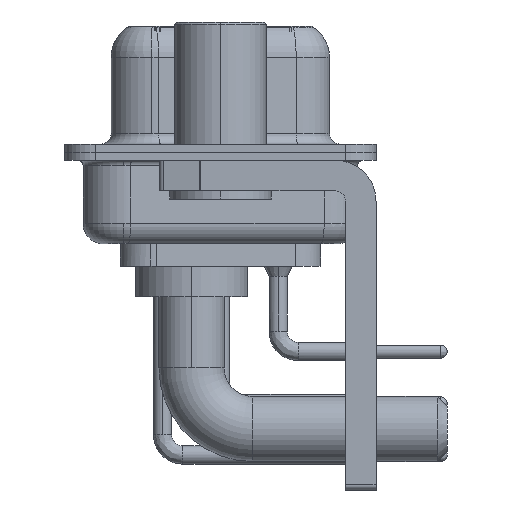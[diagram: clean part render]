
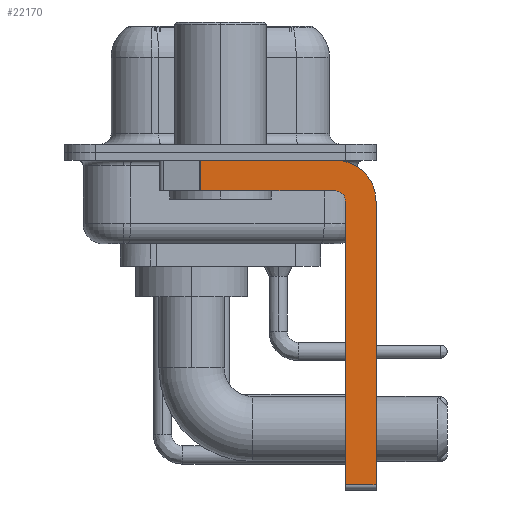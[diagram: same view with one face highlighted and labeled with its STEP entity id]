
A CAD part, left-side view. The second image highlights one B-rep face of the part: STEP entity #22170.
In plain terms, the highlighted planar face has unit normal (-1, 0, 0).
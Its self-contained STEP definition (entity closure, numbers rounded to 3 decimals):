
#495 = FACE_OUTER_BOUND ( 'NONE', #18113, .T. ) ;
#679 = DIRECTION ( 'NONE',  ( 0., 0., 1. ) ) ;
#1020 = LINE ( 'NONE', #28856, #26180 ) ;
#1079 = CARTESIAN_POINT ( 'NONE',  ( -2.9, -6.15, -16.6 ) ) ;
#1537 = DIRECTION ( 'NONE',  ( 0., 1., 0. ) ) ;
#1551 = DIRECTION ( 'NONE',  ( 1., 0., 0. ) ) ;
#1914 = DIRECTION ( 'NONE',  ( 0., 0., -1. ) ) ;
#1986 = ORIENTED_EDGE ( 'NONE', *, *, #17445, .F. ) ;
#2511 = CARTESIAN_POINT ( 'NONE',  ( -2.9, -5.65, -0.4 ) ) ;
#2996 = CARTESIAN_POINT ( 'NONE',  ( -2.9, 0.978, -1.9 ) ) ;
#3268 = VERTEX_POINT ( 'NONE', #34301 ) ;
#3313 = VERTEX_POINT ( 'NONE', #23075 ) ;
#3329 = CARTESIAN_POINT ( 'NONE',  ( -2.9, -6.15, -2.4 ) ) ;
#3332 = VECTOR ( 'NONE', #27077, 1000. ) ;
#3419 = VERTEX_POINT ( 'NONE', #7307 ) ;
#3896 = EDGE_CURVE ( 'NONE', #22963, #13782, #33438, .T. ) ;
#4553 = EDGE_CURVE ( 'NONE', #12942, #3419, #22404, .T. ) ;
#6083 = ORIENTED_EDGE ( 'NONE', *, *, #23129, .F. ) ;
#6732 = DIRECTION ( 'NONE',  ( 0., -1., 0. ) ) ;
#7307 = CARTESIAN_POINT ( 'NONE',  ( -2.9, -7.65, -16.35 ) ) ;
#7555 = ORIENTED_EDGE ( 'NONE', *, *, #3896, .T. ) ;
#8255 = DIRECTION ( 'NONE',  ( 1., 0., 0. ) ) ;
#8486 = CARTESIAN_POINT ( 'NONE',  ( -2.9, 0.978, -0.4 ) ) ;
#8625 = VERTEX_POINT ( 'NONE', #3329 ) ;
#9024 = ORIENTED_EDGE ( 'NONE', *, *, #12205, .F. ) ;
#9603 = CARTESIAN_POINT ( 'NONE',  ( -2.9, 0.978, -1.9 ) ) ;
#10071 = CARTESIAN_POINT ( 'NONE',  ( -2.9, -6.15, -16.35 ) ) ;
#10994 = AXIS2_PLACEMENT_3D ( 'NONE', #21851, #1551, #1914 ) ;
#11196 = ORIENTED_EDGE ( 'NONE', *, *, #33349, .F. ) ;
#12205 = EDGE_CURVE ( 'NONE', #3313, #3419, #35473, .T. ) ;
#12870 = AXIS2_PLACEMENT_3D ( 'NONE', #23389, #17480, #679 ) ;
#12942 = VERTEX_POINT ( 'NONE', #10071 ) ;
#13782 = VERTEX_POINT ( 'NONE', #9603 ) ;
#14178 = CARTESIAN_POINT ( 'NONE',  ( -2.9, -7.65, -2.4 ) ) ;
#15265 = VECTOR ( 'NONE', #25434, 1000. ) ;
#16901 = CIRCLE ( 'NONE', #10994, 2. ) ;
#17445 = EDGE_CURVE ( 'NONE', #3268, #13782, #35490, .T. ) ;
#17480 = DIRECTION ( 'NONE',  ( -1., 0., 0. ) ) ;
#18113 = EDGE_LOOP ( 'NONE', ( #35054, #7555, #1986, #29504, #6083, #31655, #9024, #11196 ) ) ;
#19747 = AXIS2_PLACEMENT_3D ( 'NONE', #33696, #8255, #20044 ) ;
#20044 = DIRECTION ( 'NONE',  ( 0., 0., -1. ) ) ;
#20197 = EDGE_CURVE ( 'NONE', #22963, #31110, #1020, .T. ) ;
#21851 = CARTESIAN_POINT ( 'NONE',  ( -2.9, -5.65, -2.4 ) ) ;
#22170 = ADVANCED_FACE ( 'NONE', ( #495 ), #22836, .F. ) ;
#22404 = LINE ( 'NONE', #31227, #30816 ) ;
#22836 = PLANE ( 'NONE',  #19747 ) ;
#22960 = DIRECTION ( 'NONE',  ( 0., -1., 0. ) ) ;
#22963 = VERTEX_POINT ( 'NONE', #8486 ) ;
#23075 = CARTESIAN_POINT ( 'NONE',  ( -2.9, -7.65, -2.4 ) ) ;
#23129 = EDGE_CURVE ( 'NONE', #12942, #8625, #32048, .T. ) ;
#23389 = CARTESIAN_POINT ( 'NONE',  ( -2.9, -5.65, -2.4 ) ) ;
#24905 = EDGE_CURVE ( 'NONE', #8625, #3268, #28755, .T. ) ;
#25434 = DIRECTION ( 'NONE',  ( 0., 0., -1. ) ) ;
#25980 = VECTOR ( 'NONE', #1537, 1000. ) ;
#26180 = VECTOR ( 'NONE', #6732, 1000. ) ;
#27077 = DIRECTION ( 'NONE',  ( 0., 0., 1. ) ) ;
#27882 = DIRECTION ( 'NONE',  ( 0., 0., -1. ) ) ;
#28755 = CIRCLE ( 'NONE', #12870, 0.5 ) ;
#28856 = CARTESIAN_POINT ( 'NONE',  ( -2.9, 3., -0.4 ) ) ;
#29504 = ORIENTED_EDGE ( 'NONE', *, *, #24905, .F. ) ;
#30816 = VECTOR ( 'NONE', #22960, 1000. ) ;
#31110 = VERTEX_POINT ( 'NONE', #2511 ) ;
#31227 = CARTESIAN_POINT ( 'NONE',  ( -2.9, -5.65, -16.35 ) ) ;
#31655 = ORIENTED_EDGE ( 'NONE', *, *, #4553, .T. ) ;
#32048 = LINE ( 'NONE', #1079, #3332 ) ;
#32700 = CARTESIAN_POINT ( 'NONE',  ( -2.9, -5.65, -1.9 ) ) ;
#33349 = EDGE_CURVE ( 'NONE', #31110, #3313, #16901, .T. ) ;
#33438 = LINE ( 'NONE', #2996, #36274 ) ;
#33696 = CARTESIAN_POINT ( 'NONE',  ( -2.9, -5.65, -2.4 ) ) ;
#34301 = CARTESIAN_POINT ( 'NONE',  ( -2.9, -5.65, -1.9 ) ) ;
#35054 = ORIENTED_EDGE ( 'NONE', *, *, #20197, .F. ) ;
#35473 = LINE ( 'NONE', #14178, #15265 ) ;
#35490 = LINE ( 'NONE', #32700, #25980 ) ;
#36274 = VECTOR ( 'NONE', #27882, 1000. ) ;
